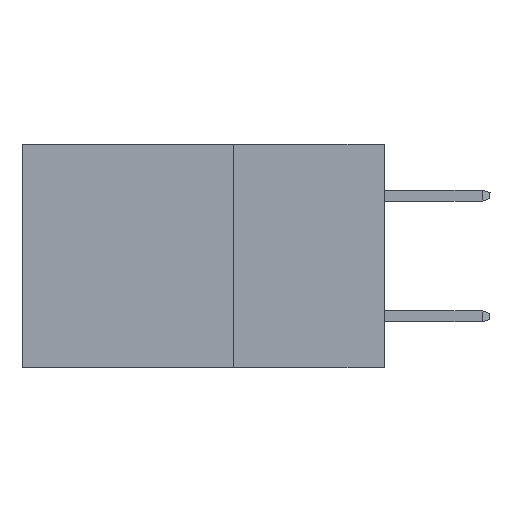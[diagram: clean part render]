
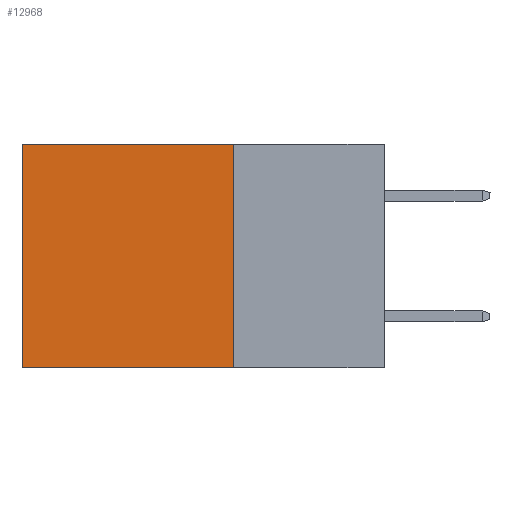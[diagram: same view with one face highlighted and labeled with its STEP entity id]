
A CAD part, left-side view. The second image highlights one B-rep face of the part: STEP entity #12968.
In plain terms, the highlighted planar face has unit normal (-1, 0, 0).
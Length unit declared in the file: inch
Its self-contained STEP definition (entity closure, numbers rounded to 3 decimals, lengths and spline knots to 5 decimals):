
#334 = DIRECTION ( 'NONE',  ( 0., 1., 0. ) ) ;
#1617 = VECTOR ( 'NONE', #5541, 39.37008 ) ;
#2428 = AXIS2_PLACEMENT_3D ( 'NONE', #10312, #26588, #12147 ) ;
#3133 = LINE ( 'NONE', #5107, #16338 ) ;
#3407 = EDGE_LOOP ( 'NONE', ( #17838, #17784, #17669, #15312 ) ) ;
#5107 = CARTESIAN_POINT ( 'NONE',  ( 0.298, 0.25, 0. ) ) ;
#5130 = CARTESIAN_POINT ( 'NONE',  ( 0.298, 0.25, -0.37 ) ) ;
#5541 = DIRECTION ( 'NONE',  ( 0., 0., -1. ) ) ;
#5881 = CARTESIAN_POINT ( 'NONE',  ( 0.298, 0.6, 0. ) ) ;
#6243 = EDGE_CURVE ( 'NONE', #22134, #8896, #3133, .T. ) ;
#7386 = LINE ( 'NONE', #17830, #1617 ) ;
#7760 = EDGE_CURVE ( 'NONE', #23702, #8156, #21142, .T. ) ;
#8156 = VERTEX_POINT ( 'NONE', #23782 ) ;
#8484 = VECTOR ( 'NONE', #11377, 39.37008 ) ;
#8832 = EDGE_CURVE ( 'NONE', #22134, #23702, #7386, .T. ) ;
#8896 = VERTEX_POINT ( 'NONE', #5881 ) ;
#10312 = CARTESIAN_POINT ( 'NONE',  ( 0.298, 0.25, 0. ) ) ;
#10444 = LINE ( 'NONE', #26154, #8484 ) ;
#11377 = DIRECTION ( 'NONE',  ( 0., 0., -1. ) ) ;
#12147 = DIRECTION ( 'NONE',  ( 0., 0., -1. ) ) ;
#12968 = ADVANCED_FACE ( 'NONE', ( #19150 ), #24611, .F. ) ;
#15312 = ORIENTED_EDGE ( 'NONE', *, *, #6243, .T. ) ;
#15599 = VECTOR ( 'NONE', #334, 39.37008 ) ;
#16338 = VECTOR ( 'NONE', #17637, 39.37008 ) ;
#17637 = DIRECTION ( 'NONE',  ( 0., 1., 0. ) ) ;
#17669 = ORIENTED_EDGE ( 'NONE', *, *, #8832, .F. ) ;
#17784 = ORIENTED_EDGE ( 'NONE', *, *, #7760, .F. ) ;
#17830 = CARTESIAN_POINT ( 'NONE',  ( 0.298, 0.25, 0. ) ) ;
#17838 = ORIENTED_EDGE ( 'NONE', *, *, #20223, .T. ) ;
#18393 = CARTESIAN_POINT ( 'NONE',  ( 0.298, 0.25, -0.37 ) ) ;
#19150 = FACE_OUTER_BOUND ( 'NONE', #3407, .T. ) ;
#20223 = EDGE_CURVE ( 'NONE', #8896, #8156, #10444, .T. ) ;
#21142 = LINE ( 'NONE', #18393, #15599 ) ;
#22134 = VERTEX_POINT ( 'NONE', #22235 ) ;
#22235 = CARTESIAN_POINT ( 'NONE',  ( 0.298, 0.25, 0. ) ) ;
#23702 = VERTEX_POINT ( 'NONE', #5130 ) ;
#23782 = CARTESIAN_POINT ( 'NONE',  ( 0.298, 0.6, -0.37 ) ) ;
#24611 = PLANE ( 'NONE',  #2428 ) ;
#26154 = CARTESIAN_POINT ( 'NONE',  ( 0.298, 0.6, 0. ) ) ;
#26588 = DIRECTION ( 'NONE',  ( 1., 0., 0. ) ) ;
